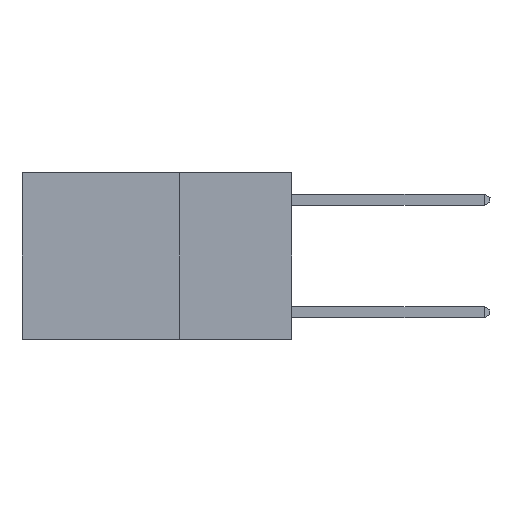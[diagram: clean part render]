
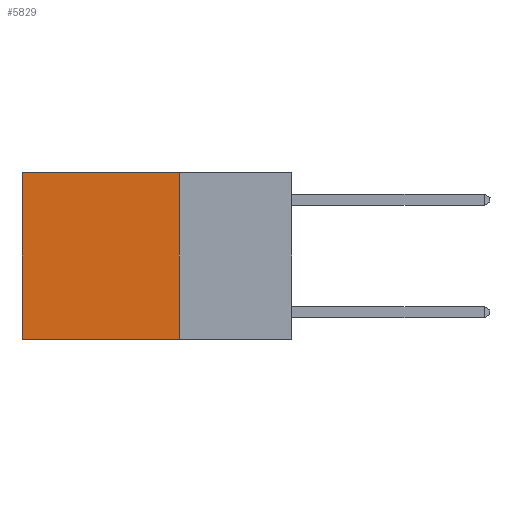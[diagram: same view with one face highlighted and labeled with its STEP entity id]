
A CAD part, left-side view. The second image highlights one B-rep face of the part: STEP entity #5829.
In plain terms, the highlighted planar face has unit normal (-1, 0, 0).
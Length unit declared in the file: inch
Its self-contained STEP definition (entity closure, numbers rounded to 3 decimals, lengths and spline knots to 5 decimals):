
#137 = VECTOR ( 'NONE', #9451, 39.37008 ) ;
#657 = DIRECTION ( 'NONE',  ( 0., 0., -1. ) ) ;
#1423 = EDGE_LOOP ( 'NONE', ( #8400, #5355, #7067, #11347 ) ) ;
#1743 = VERTEX_POINT ( 'NONE', #10984 ) ;
#2073 = CARTESIAN_POINT ( 'NONE',  ( 0.2625, 0.25, 0. ) ) ;
#2156 = DIRECTION ( 'NONE',  ( 0., 1., 0. ) ) ;
#2392 = EDGE_CURVE ( 'NONE', #1743, #9118, #10719, .T. ) ;
#2874 = AXIS2_PLACEMENT_3D ( 'NONE', #14031, #7535, #657 ) ;
#5355 = ORIENTED_EDGE ( 'NONE', *, *, #6258, .F. ) ;
#5621 = VERTEX_POINT ( 'NONE', #9320 ) ;
#5829 = ADVANCED_FACE ( 'NONE', ( #14337 ), #11876, .F. ) ;
#6258 = EDGE_CURVE ( 'NONE', #5621, #11703, #9225, .T. ) ;
#6414 = CARTESIAN_POINT ( 'NONE',  ( 0.2625, 0.6, 0. ) ) ;
#7067 = ORIENTED_EDGE ( 'NONE', *, *, #9437, .F. ) ;
#7082 = DIRECTION ( 'NONE',  ( 0., 0., -1. ) ) ;
#7247 = CARTESIAN_POINT ( 'NONE',  ( 0.2625, 0.6, -0.37 ) ) ;
#7405 = VECTOR ( 'NONE', #13171, 39.37008 ) ;
#7535 = DIRECTION ( 'NONE',  ( 1., 0., 0. ) ) ;
#8400 = ORIENTED_EDGE ( 'NONE', *, *, #14454, .T. ) ;
#9118 = VERTEX_POINT ( 'NONE', #6414 ) ;
#9225 = LINE ( 'NONE', #10559, #137 ) ;
#9320 = CARTESIAN_POINT ( 'NONE',  ( 0.2625, 0.25, -0.37 ) ) ;
#9437 = EDGE_CURVE ( 'NONE', #1743, #5621, #10634, .T. ) ;
#9451 = DIRECTION ( 'NONE',  ( 0., 1., 0. ) ) ;
#10383 = VECTOR ( 'NONE', #2156, 39.37008 ) ;
#10559 = CARTESIAN_POINT ( 'NONE',  ( 0.2625, 0.25, -0.37 ) ) ;
#10634 = LINE ( 'NONE', #2073, #7405 ) ;
#10719 = LINE ( 'NONE', #12154, #10383 ) ;
#10869 = VECTOR ( 'NONE', #7082, 39.37008 ) ;
#10984 = CARTESIAN_POINT ( 'NONE',  ( 0.2625, 0.25, 0. ) ) ;
#11347 = ORIENTED_EDGE ( 'NONE', *, *, #2392, .T. ) ;
#11703 = VERTEX_POINT ( 'NONE', #7247 ) ;
#11876 = PLANE ( 'NONE',  #2874 ) ;
#12154 = CARTESIAN_POINT ( 'NONE',  ( 0.2625, 0.25, 0. ) ) ;
#13171 = DIRECTION ( 'NONE',  ( 0., 0., -1. ) ) ;
#13440 = LINE ( 'NONE', #13603, #10869 ) ;
#13603 = CARTESIAN_POINT ( 'NONE',  ( 0.2625, 0.6, 0. ) ) ;
#14031 = CARTESIAN_POINT ( 'NONE',  ( 0.2625, 0.25, 0. ) ) ;
#14337 = FACE_OUTER_BOUND ( 'NONE', #1423, .T. ) ;
#14454 = EDGE_CURVE ( 'NONE', #9118, #11703, #13440, .T. ) ;
